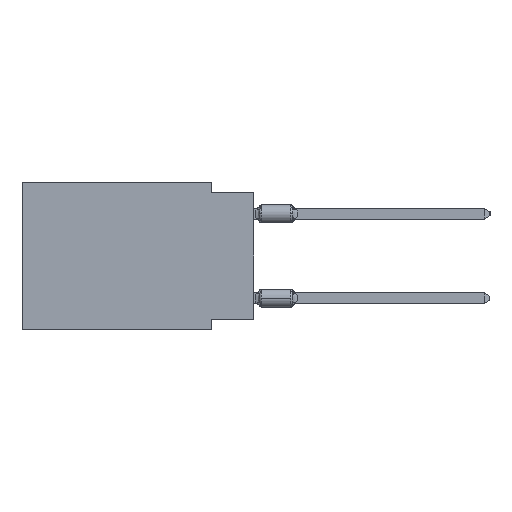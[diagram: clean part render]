
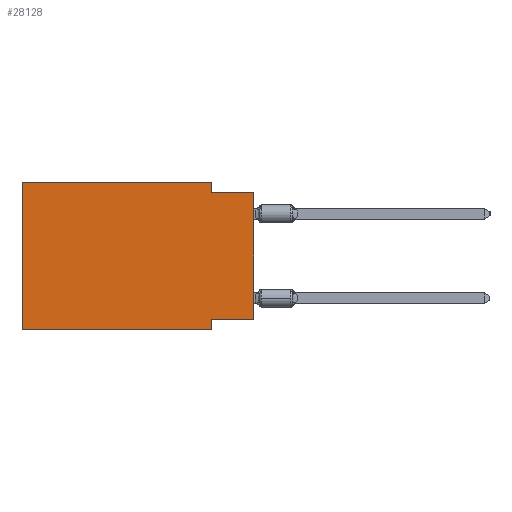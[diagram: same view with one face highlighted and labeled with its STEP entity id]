
A CAD part, left-side view. The second image highlights one B-rep face of the part: STEP entity #28128.
In plain terms, the highlighted planar face has unit normal (-1, 0, 0).
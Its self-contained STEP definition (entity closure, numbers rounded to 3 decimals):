
#107 = DIRECTION ( 'NONE',  ( 0., -1., 0. ) ) ;
#527 = CARTESIAN_POINT ( 'NONE',  ( 0., 13.97, 0. ) ) ;
#988 = LINE ( 'NONE', #527, #17569 ) ;
#1847 = EDGE_CURVE ( 'NONE', #7628, #40891, #19839, .T. ) ;
#2359 = DIRECTION ( 'NONE',  ( 0., 0., 1. ) ) ;
#2458 = VECTOR ( 'NONE', #38315, 1000. ) ;
#4577 = CARTESIAN_POINT ( 'NONE',  ( 0., 2.54, -8.255 ) ) ;
#5680 = CARTESIAN_POINT ( 'NONE',  ( 0., 2.54, -8.89 ) ) ;
#6306 = VERTEX_POINT ( 'NONE', #21159 ) ;
#7628 = VERTEX_POINT ( 'NONE', #45670 ) ;
#8251 = EDGE_CURVE ( 'NONE', #24831, #20003, #11403, .T. ) ;
#8783 = EDGE_CURVE ( 'NONE', #35065, #20003, #26232, .T. ) ;
#9103 = LINE ( 'NONE', #38380, #23612 ) ;
#9126 = EDGE_CURVE ( 'NONE', #40891, #15446, #25698, .T. ) ;
#9168 = DIRECTION ( 'NONE',  ( 0., -1., 0. ) ) ;
#10854 = ORIENTED_EDGE ( 'NONE', *, *, #8783, .F. ) ;
#11403 = LINE ( 'NONE', #25329, #41479 ) ;
#11840 = CARTESIAN_POINT ( 'NONE',  ( 0., 13.97, 0. ) ) ;
#12573 = LINE ( 'NONE', #27209, #25052 ) ;
#13330 = ORIENTED_EDGE ( 'NONE', *, *, #42847, .F. ) ;
#14042 = CARTESIAN_POINT ( 'NONE',  ( 0., 0., -0.635 ) ) ;
#15202 = CARTESIAN_POINT ( 'NONE',  ( 0., 2.54, -8.89 ) ) ;
#15420 = DIRECTION ( 'NONE',  ( 0., 0., 1. ) ) ;
#15446 = VERTEX_POINT ( 'NONE', #14042 ) ;
#17002 = CARTESIAN_POINT ( 'NONE',  ( 0., 13.97, 0. ) ) ;
#17569 = VECTOR ( 'NONE', #15420, 1000. ) ;
#17866 = VERTEX_POINT ( 'NONE', #17002 ) ;
#19532 = FACE_OUTER_BOUND ( 'NONE', #40033, .T. ) ;
#19839 = LINE ( 'NONE', #45291, #2458 ) ;
#20003 = VERTEX_POINT ( 'NONE', #5680 ) ;
#21159 = CARTESIAN_POINT ( 'NONE',  ( 0., 0., -8.255 ) ) ;
#22615 = VECTOR ( 'NONE', #9168, 1000. ) ;
#23612 = VECTOR ( 'NONE', #2359, 1000. ) ;
#23644 = ORIENTED_EDGE ( 'NONE', *, *, #45480, .F. ) ;
#24528 = CARTESIAN_POINT ( 'NONE',  ( 0., 2.54, -0.635 ) ) ;
#24778 = ORIENTED_EDGE ( 'NONE', *, *, #40701, .F. ) ;
#24831 = VERTEX_POINT ( 'NONE', #44187 ) ;
#25052 = VECTOR ( 'NONE', #41855, 1000. ) ;
#25329 = CARTESIAN_POINT ( 'NONE',  ( 0., 13.97, -8.89 ) ) ;
#25698 = LINE ( 'NONE', #29063, #28514 ) ;
#26232 = LINE ( 'NONE', #15202, #32318 ) ;
#26699 = LINE ( 'NONE', #30782, #22615 ) ;
#27209 = CARTESIAN_POINT ( 'NONE',  ( 0., 0., -8.255 ) ) ;
#28128 = ADVANCED_FACE ( 'NONE', ( #19532 ), #38245, .F. ) ;
#28514 = VECTOR ( 'NONE', #32902, 1000. ) ;
#29063 = CARTESIAN_POINT ( 'NONE',  ( 0., 0., -0.635 ) ) ;
#30378 = ORIENTED_EDGE ( 'NONE', *, *, #44803, .T. ) ;
#30782 = CARTESIAN_POINT ( 'NONE',  ( 0., 13.97, 0. ) ) ;
#32318 = VECTOR ( 'NONE', #44244, 1000. ) ;
#32902 = DIRECTION ( 'NONE',  ( 0., -1., 0. ) ) ;
#33930 = DIRECTION ( 'NONE',  ( 0., 0., -1. ) ) ;
#35065 = VERTEX_POINT ( 'NONE', #4577 ) ;
#35231 = ORIENTED_EDGE ( 'NONE', *, *, #9126, .F. ) ;
#35596 = ORIENTED_EDGE ( 'NONE', *, *, #8251, .T. ) ;
#37805 = AXIS2_PLACEMENT_3D ( 'NONE', #11840, #41385, #33930 ) ;
#38245 = PLANE ( 'NONE',  #37805 ) ;
#38315 = DIRECTION ( 'NONE',  ( 0., 0., -1. ) ) ;
#38380 = CARTESIAN_POINT ( 'NONE',  ( 0., 0., 0. ) ) ;
#40033 = EDGE_LOOP ( 'NONE', ( #30378, #35231, #47108, #24778, #23644, #35596, #10854, #13330 ) ) ;
#40701 = EDGE_CURVE ( 'NONE', #17866, #7628, #26699, .T. ) ;
#40891 = VERTEX_POINT ( 'NONE', #24528 ) ;
#41385 = DIRECTION ( 'NONE',  ( 1., 0., 0. ) ) ;
#41479 = VECTOR ( 'NONE', #107, 1000. ) ;
#41855 = DIRECTION ( 'NONE',  ( 0., 1., 0. ) ) ;
#42847 = EDGE_CURVE ( 'NONE', #6306, #35065, #12573, .T. ) ;
#44187 = CARTESIAN_POINT ( 'NONE',  ( 0., 13.97, -8.89 ) ) ;
#44244 = DIRECTION ( 'NONE',  ( 0., 0., -1. ) ) ;
#44803 = EDGE_CURVE ( 'NONE', #6306, #15446, #9103, .T. ) ;
#45291 = CARTESIAN_POINT ( 'NONE',  ( 0., 2.54, 0. ) ) ;
#45480 = EDGE_CURVE ( 'NONE', #24831, #17866, #988, .T. ) ;
#45670 = CARTESIAN_POINT ( 'NONE',  ( 0., 2.54, 0. ) ) ;
#47108 = ORIENTED_EDGE ( 'NONE', *, *, #1847, .F. ) ;
